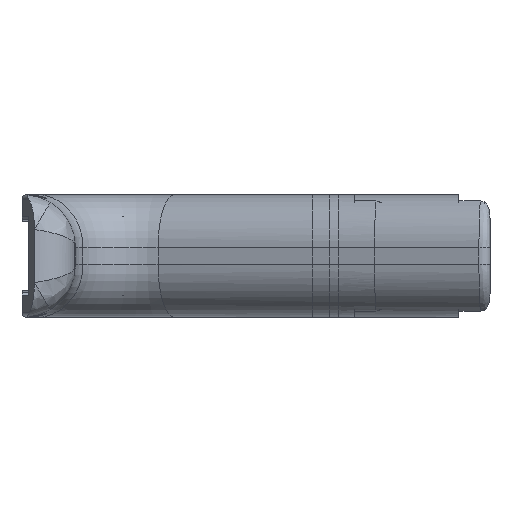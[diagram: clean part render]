
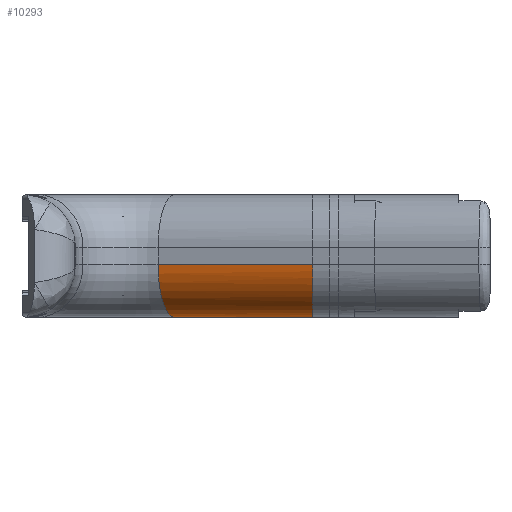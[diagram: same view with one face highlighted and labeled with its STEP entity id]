
A CAD part, left-side view. The second image highlights one B-rep face of the part: STEP entity #10293.
In plain terms, the highlighted cylindrical face has radius 12.5 mm (diameter 25 mm), a partial arc.
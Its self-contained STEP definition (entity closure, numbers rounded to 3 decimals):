
#253=ELLIPSE('',#10782,13.143,12.5);
#479=CYLINDRICAL_SURFACE('',#11105,12.5);
#893=FACE_OUTER_BOUND('',#1458,.T.);
#1458=EDGE_LOOP('',(#8530,#8531,#8532,#8533));
#1795=CIRCLE('',#10934,12.5);
#2236=LINE('',#15782,#3302);
#2585=LINE('',#17901,#3651);
#3302=VECTOR('',#12310,10.);
#3651=VECTOR('',#13273,10.);
#4336=VERTEX_POINT('',#15584);
#4341=VERTEX_POINT('',#15594);
#4377=VERTEX_POINT('',#15781);
#4511=VERTEX_POINT('',#17314);
#5462=EDGE_CURVE('',#4341,#4336,#253,.T.);
#5505=EDGE_CURVE('',#4377,#4336,#2236,.T.);
#5733=EDGE_CURVE('',#4511,#4377,#1795,.T.);
#6024=EDGE_CURVE('',#4341,#4511,#2585,.T.);
#8530=ORIENTED_EDGE('',*,*,#5462,.F.);
#8531=ORIENTED_EDGE('',*,*,#6024,.T.);
#8532=ORIENTED_EDGE('',*,*,#5733,.T.);
#8533=ORIENTED_EDGE('',*,*,#5505,.T.);
#10293=ADVANCED_FACE('',(#893),#479,.T.);
#10782=AXIS2_PLACEMENT_3D('',#15596,#12256,#12257);
#10934=AXIS2_PLACEMENT_3D('',#17315,#12690,#12691);
#11105=AXIS2_PLACEMENT_3D('',#17900,#13271,#13272);
#12256=DIRECTION('center_axis',(0.,-1.,0.));
#12257=DIRECTION('ref_axis',(-1.,0.,0.));
#12310=DIRECTION('',(-0.309,-0.951,0.));
#12690=DIRECTION('center_axis',(-0.309,-0.951,0.));
#12691=DIRECTION('ref_axis',(-0.951,0.309,0.));
#13271=DIRECTION('center_axis',(-0.309,-0.951,0.));
#13272=DIRECTION('ref_axis',(-0.672,0.219,-0.707));
#13273=DIRECTION('',(0.309,0.951,0.));
#15584=CARTESIAN_POINT('',(-64.797,-19.479,-34.));
#15594=CARTESIAN_POINT('',(-77.94,-19.479,-21.5));
#15596=CARTESIAN_POINT('Origin',(-64.797,-19.479,-21.5));
#15781=CARTESIAN_POINT('',(-54.134,13.337,-34.));
#15782=CARTESIAN_POINT('',(-50.012,26.025,-34.));
#17314=CARTESIAN_POINT('',(-66.022,17.2,-21.5));
#17315=CARTESIAN_POINT('Origin',(-54.134,13.337,-21.5));
#17900=CARTESIAN_POINT('Origin',(-50.012,26.025,-21.5));
#17901=CARTESIAN_POINT('',(-61.9,29.887,-21.5));
